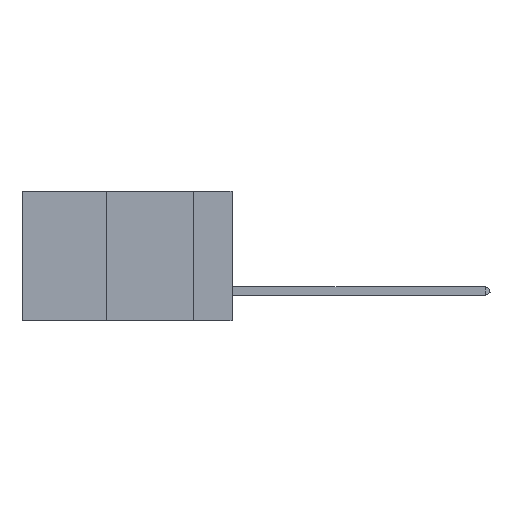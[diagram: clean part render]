
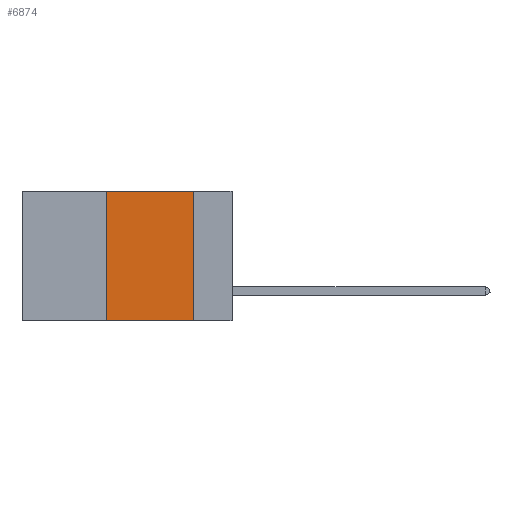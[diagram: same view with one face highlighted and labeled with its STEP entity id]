
A CAD part, left-side view. The second image highlights one B-rep face of the part: STEP entity #6874.
In plain terms, the highlighted planar face has unit normal (-1, 0, 0).
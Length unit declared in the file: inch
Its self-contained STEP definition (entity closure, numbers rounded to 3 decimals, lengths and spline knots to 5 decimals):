
#549 = EDGE_CURVE ( 'NONE', #3299, #14356, #9749, .T. ) ;
#1451 = LINE ( 'NONE', #5951, #3384 ) ;
#2484 = DIRECTION ( 'NONE',  ( 0., -1., 0. ) ) ;
#2740 = LINE ( 'NONE', #11715, #2958 ) ;
#2917 = DIRECTION ( 'NONE',  ( 0., 0., -1. ) ) ;
#2958 = VECTOR ( 'NONE', #17322, 39.37008 ) ;
#3299 = VERTEX_POINT ( 'NONE', #15934 ) ;
#3384 = VECTOR ( 'NONE', #4633, 39.37008 ) ;
#4074 = CARTESIAN_POINT ( 'NONE',  ( 0., 0.11, 0. ) ) ;
#4077 = AXIS2_PLACEMENT_3D ( 'NONE', #15198, #16645, #2917 ) ;
#4633 = DIRECTION ( 'NONE',  ( 0., 0., -1. ) ) ;
#4697 = ORIENTED_EDGE ( 'NONE', *, *, #12426, .T. ) ;
#5419 = ORIENTED_EDGE ( 'NONE', *, *, #9107, .F. ) ;
#5951 = CARTESIAN_POINT ( 'NONE',  ( 0., 0.11, 0. ) ) ;
#6079 = VECTOR ( 'NONE', #6953, 39.37008 ) ;
#6324 = LINE ( 'NONE', #10872, #12415 ) ;
#6874 = ADVANCED_FACE ( 'NONE', ( #9307 ), #16587, .F. ) ;
#6953 = DIRECTION ( 'NONE',  ( 0., 0., 1. ) ) ;
#9107 = EDGE_CURVE ( 'NONE', #14356, #15716, #2740, .T. ) ;
#9134 = ORIENTED_EDGE ( 'NONE', *, *, #549, .F. ) ;
#9307 = FACE_OUTER_BOUND ( 'NONE', #11617, .T. ) ;
#9749 = LINE ( 'NONE', #9819, #6079 ) ;
#9819 = CARTESIAN_POINT ( 'NONE',  ( 0., 0.36, 0. ) ) ;
#10691 = CARTESIAN_POINT ( 'NONE',  ( 0., 0.11, -0.37 ) ) ;
#10872 = CARTESIAN_POINT ( 'NONE',  ( 0., 0.6, -0.37 ) ) ;
#11617 = EDGE_LOOP ( 'NONE', ( #14331, #5419, #9134, #4697 ) ) ;
#11715 = CARTESIAN_POINT ( 'NONE',  ( 0., 0.6, 0. ) ) ;
#11828 = VERTEX_POINT ( 'NONE', #10691 ) ;
#12415 = VECTOR ( 'NONE', #2484, 39.37008 ) ;
#12426 = EDGE_CURVE ( 'NONE', #3299, #11828, #6324, .T. ) ;
#14331 = ORIENTED_EDGE ( 'NONE', *, *, #16625, .F. ) ;
#14356 = VERTEX_POINT ( 'NONE', #15812 ) ;
#15198 = CARTESIAN_POINT ( 'NONE',  ( 0., 0.6, 0. ) ) ;
#15716 = VERTEX_POINT ( 'NONE', #4074 ) ;
#15812 = CARTESIAN_POINT ( 'NONE',  ( 0., 0.36, 0. ) ) ;
#15934 = CARTESIAN_POINT ( 'NONE',  ( 0., 0.36, -0.37 ) ) ;
#16587 = PLANE ( 'NONE',  #4077 ) ;
#16625 = EDGE_CURVE ( 'NONE', #15716, #11828, #1451, .T. ) ;
#16645 = DIRECTION ( 'NONE',  ( 1., 0., 0. ) ) ;
#17322 = DIRECTION ( 'NONE',  ( 0., -1., 0. ) ) ;
